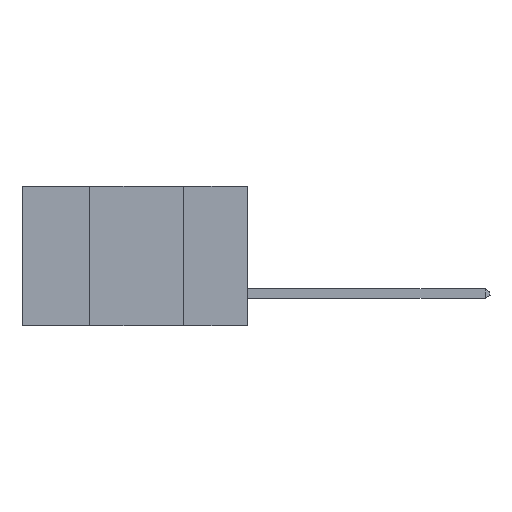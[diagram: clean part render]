
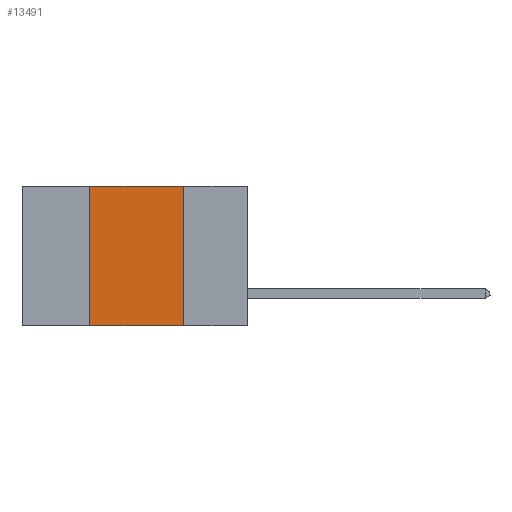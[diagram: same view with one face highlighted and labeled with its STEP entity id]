
A CAD part, left-side view. The second image highlights one B-rep face of the part: STEP entity #13491.
In plain terms, the highlighted planar face has unit normal (-1, 0, 0).
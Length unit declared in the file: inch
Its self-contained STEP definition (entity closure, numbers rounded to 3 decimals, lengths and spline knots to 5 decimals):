
#406 = CARTESIAN_POINT ( 'NONE',  ( 0., 0.42, 0. ) ) ;
#2755 = CARTESIAN_POINT ( 'NONE',  ( 0., 0.6, -0.37 ) ) ;
#2882 = LINE ( 'NONE', #21625, #21507 ) ;
#4076 = DIRECTION ( 'NONE',  ( 0., 0., -1. ) ) ;
#4524 = EDGE_LOOP ( 'NONE', ( #23199, #5049, #11036, #9038 ) ) ;
#4868 = DIRECTION ( 'NONE',  ( 0., -1., 0. ) ) ;
#5049 = ORIENTED_EDGE ( 'NONE', *, *, #20232, .F. ) ;
#5441 = DIRECTION ( 'NONE',  ( 0., 0., -1. ) ) ;
#6020 = EDGE_CURVE ( 'NONE', #10256, #9337, #6796, .T. ) ;
#6053 = PLANE ( 'NONE',  #22304 ) ;
#6279 = LINE ( 'NONE', #8138, #13060 ) ;
#6662 = CARTESIAN_POINT ( 'NONE',  ( 0., 0.42, 0. ) ) ;
#6796 = LINE ( 'NONE', #2755, #18108 ) ;
#8138 = CARTESIAN_POINT ( 'NONE',  ( 0., 0.6, 0. ) ) ;
#9038 = ORIENTED_EDGE ( 'NONE', *, *, #6020, .T. ) ;
#9337 = VERTEX_POINT ( 'NONE', #22930 ) ;
#9935 = CARTESIAN_POINT ( 'NONE',  ( 0., 0.17, 0. ) ) ;
#10256 = VERTEX_POINT ( 'NONE', #14800 ) ;
#10863 = EDGE_CURVE ( 'NONE', #10256, #19104, #19553, .T. ) ;
#11036 = ORIENTED_EDGE ( 'NONE', *, *, #10863, .F. ) ;
#11126 = EDGE_CURVE ( 'NONE', #12341, #9337, #2882, .T. ) ;
#11611 = DIRECTION ( 'NONE',  ( 0., -1., 0. ) ) ;
#11641 = VECTOR ( 'NONE', #18401, 39.37008 ) ;
#12341 = VERTEX_POINT ( 'NONE', #9935 ) ;
#13060 = VECTOR ( 'NONE', #11611, 39.37008 ) ;
#13491 = ADVANCED_FACE ( 'NONE', ( #15464 ), #6053, .F. ) ;
#14800 = CARTESIAN_POINT ( 'NONE',  ( 0., 0.42, -0.37 ) ) ;
#14894 = CARTESIAN_POINT ( 'NONE',  ( 0., 0.6, 0. ) ) ;
#15464 = FACE_OUTER_BOUND ( 'NONE', #4524, .T. ) ;
#18108 = VECTOR ( 'NONE', #4868, 39.37008 ) ;
#18401 = DIRECTION ( 'NONE',  ( 0., 0., 1. ) ) ;
#19104 = VERTEX_POINT ( 'NONE', #6662 ) ;
#19553 = LINE ( 'NONE', #406, #11641 ) ;
#20232 = EDGE_CURVE ( 'NONE', #19104, #12341, #6279, .T. ) ;
#20429 = DIRECTION ( 'NONE',  ( 1., 0., 0. ) ) ;
#21507 = VECTOR ( 'NONE', #5441, 39.37008 ) ;
#21625 = CARTESIAN_POINT ( 'NONE',  ( 0., 0.17, 0. ) ) ;
#22304 = AXIS2_PLACEMENT_3D ( 'NONE', #14894, #20429, #4076 ) ;
#22930 = CARTESIAN_POINT ( 'NONE',  ( 0., 0.17, -0.37 ) ) ;
#23199 = ORIENTED_EDGE ( 'NONE', *, *, #11126, .F. ) ;
